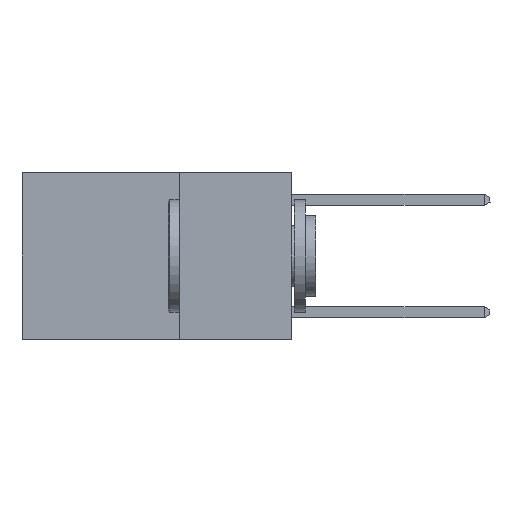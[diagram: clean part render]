
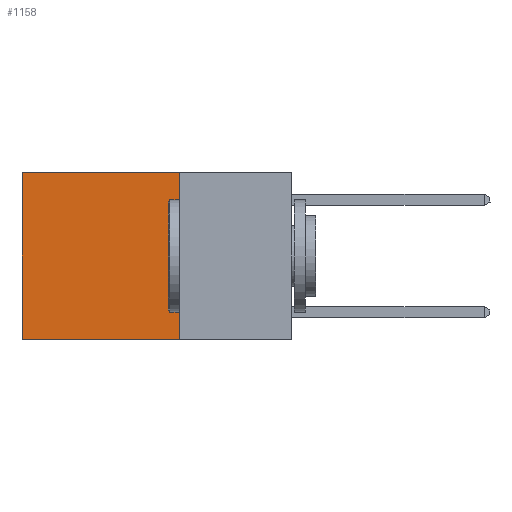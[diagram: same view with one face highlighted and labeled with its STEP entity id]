
A CAD part, left-side view. The second image highlights one B-rep face of the part: STEP entity #1158.
In plain terms, the highlighted planar face has unit normal (-1, 0, 0).
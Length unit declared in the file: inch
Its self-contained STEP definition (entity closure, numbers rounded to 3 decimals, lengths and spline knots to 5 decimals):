
#686 = CARTESIAN_POINT ( 'NONE',  ( 0.2625, 0.25, 0. ) ) ;
#1113 = DIRECTION ( 'NONE',  ( 0., 0., -1. ) ) ;
#1125 = EDGE_CURVE ( 'NONE', #3205, #10820, #8578, .T. ) ;
#1158 = ADVANCED_FACE ( 'NONE', ( #8168 ), #11620, .F. ) ;
#1174 = CARTESIAN_POINT ( 'NONE',  ( 0.2625, 0.25, 0. ) ) ;
#1291 = VERTEX_POINT ( 'NONE', #8687 ) ;
#2142 = CARTESIAN_POINT ( 'NONE',  ( 0.2625, 0.6, 0. ) ) ;
#2263 = EDGE_CURVE ( 'NONE', #6364, #3205, #8858, .T. ) ;
#2281 = ORIENTED_EDGE ( 'NONE', *, *, #2263, .T. ) ;
#2559 = CARTESIAN_POINT ( 'NONE',  ( 0.2625, 0.6, 0. ) ) ;
#2650 = AXIS2_PLACEMENT_3D ( 'NONE', #8919, #6440, #14712 ) ;
#2734 = VECTOR ( 'NONE', #15850, 39.37008 ) ;
#3205 = VERTEX_POINT ( 'NONE', #2142 ) ;
#5241 = VECTOR ( 'NONE', #9463, 39.37008 ) ;
#5506 = VECTOR ( 'NONE', #7886, 39.37008 ) ;
#6364 = VERTEX_POINT ( 'NONE', #12464 ) ;
#6440 = DIRECTION ( 'NONE',  ( 1., 0., 0. ) ) ;
#7294 = EDGE_LOOP ( 'NONE', ( #9574, #8646, #12013, #2281 ) ) ;
#7886 = DIRECTION ( 'NONE',  ( 0., 1., 0. ) ) ;
#8168 = FACE_OUTER_BOUND ( 'NONE', #7294, .T. ) ;
#8570 = EDGE_CURVE ( 'NONE', #1291, #10820, #9467, .T. ) ;
#8578 = LINE ( 'NONE', #2559, #5241 ) ;
#8646 = ORIENTED_EDGE ( 'NONE', *, *, #8570, .F. ) ;
#8687 = CARTESIAN_POINT ( 'NONE',  ( 0.2625, 0.25, -0.37 ) ) ;
#8858 = LINE ( 'NONE', #686, #5506 ) ;
#8919 = CARTESIAN_POINT ( 'NONE',  ( 0.2625, 0.25, 0. ) ) ;
#9463 = DIRECTION ( 'NONE',  ( 0., 0., -1. ) ) ;
#9467 = LINE ( 'NONE', #12158, #2734 ) ;
#9574 = ORIENTED_EDGE ( 'NONE', *, *, #1125, .T. ) ;
#10323 = CARTESIAN_POINT ( 'NONE',  ( 0.2625, 0.6, -0.37 ) ) ;
#10799 = VECTOR ( 'NONE', #1113, 39.37008 ) ;
#10820 = VERTEX_POINT ( 'NONE', #10323 ) ;
#11620 = PLANE ( 'NONE',  #2650 ) ;
#12013 = ORIENTED_EDGE ( 'NONE', *, *, #13114, .F. ) ;
#12158 = CARTESIAN_POINT ( 'NONE',  ( 0.2625, 0.25, -0.37 ) ) ;
#12464 = CARTESIAN_POINT ( 'NONE',  ( 0.2625, 0.25, 0. ) ) ;
#13114 = EDGE_CURVE ( 'NONE', #6364, #1291, #14094, .T. ) ;
#14094 = LINE ( 'NONE', #1174, #10799 ) ;
#14712 = DIRECTION ( 'NONE',  ( 0., 0., -1. ) ) ;
#15850 = DIRECTION ( 'NONE',  ( 0., 1., 0. ) ) ;
